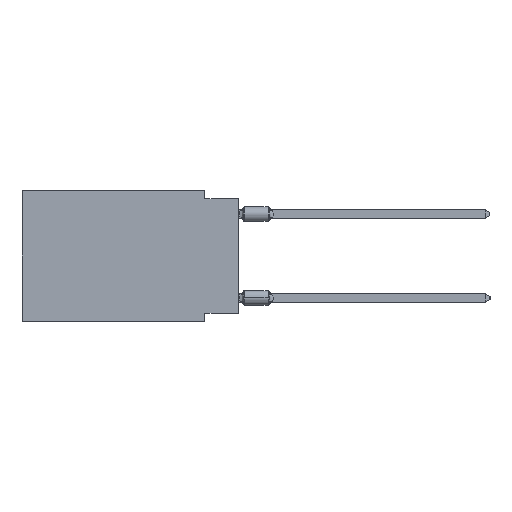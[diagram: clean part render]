
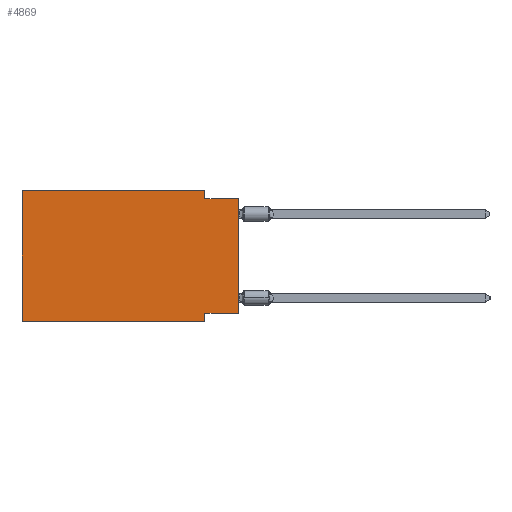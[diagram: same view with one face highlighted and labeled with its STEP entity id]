
A CAD part, left-side view. The second image highlights one B-rep face of the part: STEP entity #4869.
In plain terms, the highlighted planar face has unit normal (-1, 0, 0).
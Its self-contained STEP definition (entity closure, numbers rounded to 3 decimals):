
#154 = ORIENTED_EDGE ( 'NONE', *, *, #33433, .T. ) ;
#500 = DIRECTION ( 'NONE',  ( 0., 0., -1. ) ) ;
#659 = CARTESIAN_POINT ( 'NONE',  ( 0., 2.54, -9.271 ) ) ;
#917 = VERTEX_POINT ( 'NONE', #38026 ) ;
#933 = CARTESIAN_POINT ( 'NONE',  ( 0., 16.383, 0. ) ) ;
#1133 = LINE ( 'NONE', #933, #40321 ) ;
#2387 = VERTEX_POINT ( 'NONE', #39880 ) ;
#2639 = CARTESIAN_POINT ( 'NONE',  ( 0., 0., -0.635 ) ) ;
#4869 = ADVANCED_FACE ( 'NONE', ( #20705 ), #7639, .F. ) ;
#5135 = DIRECTION ( 'NONE',  ( 1., 0., 0. ) ) ;
#5326 = EDGE_CURVE ( 'NONE', #40008, #35619, #32904, .T. ) ;
#7234 = CARTESIAN_POINT ( 'NONE',  ( 0., 2.54, 0. ) ) ;
#7289 = VERTEX_POINT ( 'NONE', #659 ) ;
#7639 = PLANE ( 'NONE',  #21441 ) ;
#7793 = DIRECTION ( 'NONE',  ( 0., -1., 0. ) ) ;
#8979 = CARTESIAN_POINT ( 'NONE',  ( 0., 0., 0. ) ) ;
#9997 = DIRECTION ( 'NONE',  ( 0., 1., 0. ) ) ;
#10919 = CARTESIAN_POINT ( 'NONE',  ( 0., 16.383, -9.906 ) ) ;
#10993 = ORIENTED_EDGE ( 'NONE', *, *, #33377, .F. ) ;
#11999 = VERTEX_POINT ( 'NONE', #27958 ) ;
#12486 = LINE ( 'NONE', #24947, #22968 ) ;
#13630 = EDGE_CURVE ( 'NONE', #40008, #11999, #12486, .T. ) ;
#13813 = EDGE_CURVE ( 'NONE', #2387, #7289, #14136, .T. ) ;
#14136 = LINE ( 'NONE', #26799, #35566 ) ;
#14716 = LINE ( 'NONE', #2639, #35990 ) ;
#15999 = EDGE_LOOP ( 'NONE', ( #154, #34655, #21067, #30185, #24794, #24902, #10993, #29709 ) ) ;
#16747 = VERTEX_POINT ( 'NONE', #19670 ) ;
#16999 = CARTESIAN_POINT ( 'NONE',  ( 0., 16.383, 0. ) ) ;
#17409 = DIRECTION ( 'NONE',  ( 0., 0., -1. ) ) ;
#18734 = LINE ( 'NONE', #25177, #23463 ) ;
#18810 = VECTOR ( 'NONE', #21643, 1000. ) ;
#19670 = CARTESIAN_POINT ( 'NONE',  ( 0., 0., -0.635 ) ) ;
#20073 = EDGE_CURVE ( 'NONE', #36617, #917, #35559, .T. ) ;
#20705 = FACE_OUTER_BOUND ( 'NONE', #15999, .T. ) ;
#21067 = ORIENTED_EDGE ( 'NONE', *, *, #20073, .F. ) ;
#21441 = AXIS2_PLACEMENT_3D ( 'NONE', #16999, #5135, #17409 ) ;
#21643 = DIRECTION ( 'NONE',  ( 0., 0., 1. ) ) ;
#22968 = VECTOR ( 'NONE', #25160, 1000. ) ;
#23229 = VECTOR ( 'NONE', #500, 1000. ) ;
#23463 = VECTOR ( 'NONE', #40694, 1000. ) ;
#24048 = DIRECTION ( 'NONE',  ( 0., -1., 0. ) ) ;
#24794 = ORIENTED_EDGE ( 'NONE', *, *, #13630, .F. ) ;
#24902 = ORIENTED_EDGE ( 'NONE', *, *, #5326, .T. ) ;
#24947 = CARTESIAN_POINT ( 'NONE',  ( 0., 16.383, 0. ) ) ;
#25160 = DIRECTION ( 'NONE',  ( 0., 0., 1. ) ) ;
#25177 = CARTESIAN_POINT ( 'NONE',  ( 0., 2.54, -9.906 ) ) ;
#26057 = EDGE_CURVE ( 'NONE', #11999, #36617, #1133, .T. ) ;
#26799 = CARTESIAN_POINT ( 'NONE',  ( 0., 0., -9.271 ) ) ;
#27958 = CARTESIAN_POINT ( 'NONE',  ( 0., 16.383, 0. ) ) ;
#29709 = ORIENTED_EDGE ( 'NONE', *, *, #13813, .F. ) ;
#29788 = DIRECTION ( 'NONE',  ( 0., -1., 0. ) ) ;
#30185 = ORIENTED_EDGE ( 'NONE', *, *, #26057, .F. ) ;
#32402 = EDGE_CURVE ( 'NONE', #917, #16747, #14716, .T. ) ;
#32904 = LINE ( 'NONE', #10919, #39350 ) ;
#33377 = EDGE_CURVE ( 'NONE', #7289, #35619, #18734, .T. ) ;
#33433 = EDGE_CURVE ( 'NONE', #2387, #16747, #37178, .T. ) ;
#34655 = ORIENTED_EDGE ( 'NONE', *, *, #32402, .F. ) ;
#35559 = LINE ( 'NONE', #38663, #23229 ) ;
#35566 = VECTOR ( 'NONE', #9997, 1000. ) ;
#35619 = VERTEX_POINT ( 'NONE', #40499 ) ;
#35791 = CARTESIAN_POINT ( 'NONE',  ( 0., 16.383, -9.906 ) ) ;
#35990 = VECTOR ( 'NONE', #24048, 1000. ) ;
#36617 = VERTEX_POINT ( 'NONE', #7234 ) ;
#37178 = LINE ( 'NONE', #8979, #18810 ) ;
#38026 = CARTESIAN_POINT ( 'NONE',  ( 0., 2.54, -0.635 ) ) ;
#38663 = CARTESIAN_POINT ( 'NONE',  ( 0., 2.54, 0. ) ) ;
#39350 = VECTOR ( 'NONE', #7793, 1000. ) ;
#39880 = CARTESIAN_POINT ( 'NONE',  ( 0., 0., -9.271 ) ) ;
#40008 = VERTEX_POINT ( 'NONE', #35791 ) ;
#40321 = VECTOR ( 'NONE', #29788, 1000. ) ;
#40499 = CARTESIAN_POINT ( 'NONE',  ( 0., 2.54, -9.906 ) ) ;
#40694 = DIRECTION ( 'NONE',  ( 0., 0., -1. ) ) ;
